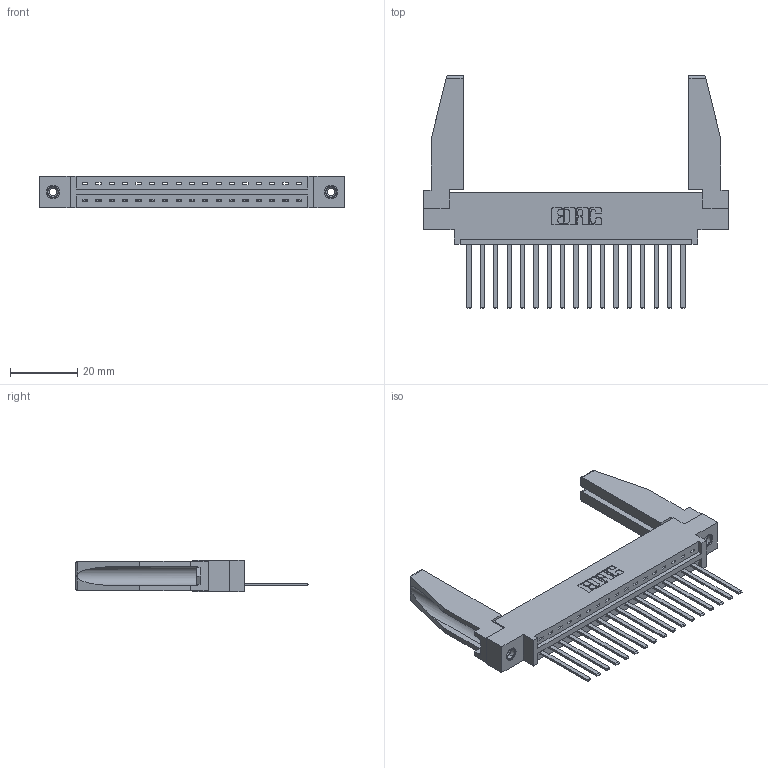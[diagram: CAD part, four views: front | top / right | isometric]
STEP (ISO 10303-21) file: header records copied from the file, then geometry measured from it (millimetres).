
FILE_DESCRIPTION (( 'STEP AP203' ), '1' );
FILE_NAME ('337-017-544-678.STEP', '2019-09-28T19:18:17', ( '' ), ( '' ), 'SwSTEP 2.0', 'SolidWorks 2016', '' );
FILE_SCHEMA (( 'CONFIG_CONTROL_DESIGN' ));
Length unit declared in the file: inch
Products named in the file (5): 345-250-001_345-250-001-102; 337-017-544-678; 345-292-001_345-293-144; 307-220-078; 337 Part_0.170 Offset - 0.156 Dia-TI
Assembly tree (22 placements, depth 2):
  337-017-544-678
    337 Part_0.170 Offset - 0.156 Dia-TI
    345-292-001_345-293-144  x17
    345-250-001_345-250-001-102  x2
    307-220-078  x2
Bounding box: 90.37 x 69.09 x 9.4 mm (x, y, z)
Volume: 13152.6 mm3; surface area: 13907 mm2
Topology: 22 solids, 22 shells, 1200 faces, 3543 edges, 2330 vertices
Faces by surface type: plane 872, cylinder 312, cone 12, torus 4
Entity records: 18258 total; most frequent: CARTESIAN_POINT 3171, ORIENTED_EDGE 3080, DIRECTION 2726, EDGE_CURVE 1540, LINE 1378, VECTOR 1378, VERTEX_POINT 1020, AXIS2_PLACEMENT_3D 674
